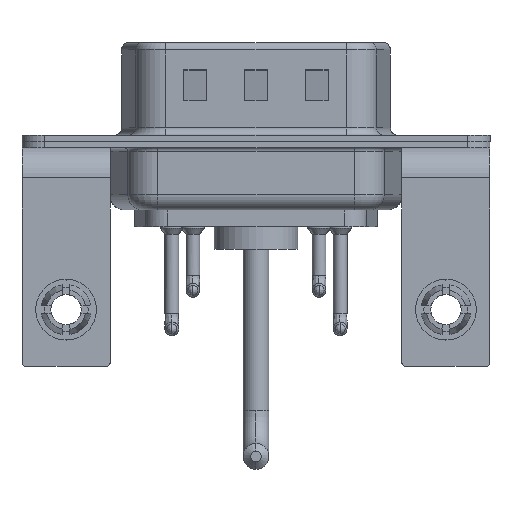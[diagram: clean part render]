
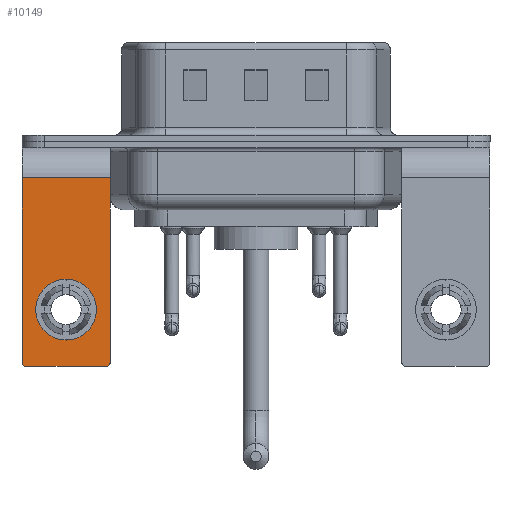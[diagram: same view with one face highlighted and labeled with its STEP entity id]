
A CAD part, front view. The second image highlights one B-rep face of the part: STEP entity #10149.
In plain terms, the highlighted planar face has unit normal (0, -1, 0).
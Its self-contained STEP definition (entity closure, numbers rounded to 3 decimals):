
#185 = DIRECTION ( 'NONE',  ( 0., 0., 1. ) ) ;
#864 = FACE_OUTER_BOUND ( 'NONE', #9699, .T. ) ;
#1735 = DIRECTION ( 'NONE',  ( 0., -1., 0. ) ) ;
#1740 = CARTESIAN_POINT ( 'NONE',  ( 0., -6.25, -11.07 ) ) ;
#1977 = VECTOR ( 'NONE', #4359, 1000. ) ;
#2109 = CARTESIAN_POINT ( 'NONE',  ( -2.65, -6.25, -14.8 ) ) ;
#2122 = DIRECTION ( 'NONE',  ( 0., 1., 0. ) ) ;
#2228 = VECTOR ( 'NONE', #6798, 1000. ) ;
#2247 = EDGE_CURVE ( 'NONE', #16355, #16900, #10989, .T. ) ;
#2508 = CARTESIAN_POINT ( 'NONE',  ( -2.65, -6.25, -14.55 ) ) ;
#2627 = DIRECTION ( 'NONE',  ( 0., 0., 1. ) ) ;
#2643 = CARTESIAN_POINT ( 'NONE',  ( 2.65, -6.25, -14.8 ) ) ;
#2855 = EDGE_CURVE ( 'NONE', #8489, #16174, #4055, .T. ) ;
#3409 = DIRECTION ( 'NONE',  ( 0., 0., 1. ) ) ;
#3524 = VERTEX_POINT ( 'NONE', #2643 ) ;
#4055 = CIRCLE ( 'NONE', #6878, 2. ) ;
#4086 = DIRECTION ( 'NONE',  ( 0., -1., 0. ) ) ;
#4359 = DIRECTION ( 'NONE',  ( -1., 0., 0. ) ) ;
#4450 = DIRECTION ( 'NONE',  ( -1., 0., 0. ) ) ;
#4702 = CARTESIAN_POINT ( 'NONE',  ( -2.9, -6.25, -14.55 ) ) ;
#4952 = VERTEX_POINT ( 'NONE', #2109 ) ;
#5568 = CIRCLE ( 'NONE', #12642, 2. ) ;
#5729 = CARTESIAN_POINT ( 'NONE',  ( -2.9, -6.25, -2.4 ) ) ;
#6011 = LINE ( 'NONE', #12774, #1977 ) ;
#6091 = ORIENTED_EDGE ( 'NONE', *, *, #17905, .F. ) ;
#6798 = DIRECTION ( 'NONE',  ( 0., 0., -1. ) ) ;
#6839 = DIRECTION ( 'NONE',  ( 0., 0., 1. ) ) ;
#6878 = AXIS2_PLACEMENT_3D ( 'NONE', #12440, #2122, #9328 ) ;
#7045 = EDGE_CURVE ( 'NONE', #16174, #8489, #5568, .T. ) ;
#7356 = CIRCLE ( 'NONE', #14770, 0.25 ) ;
#7402 = AXIS2_PLACEMENT_3D ( 'NONE', #2508, #4086, #2627 ) ;
#7835 = DIRECTION ( 'NONE',  ( 0., 1., 0. ) ) ;
#8130 = ORIENTED_EDGE ( 'NONE', *, *, #9040, .T. ) ;
#8357 = LINE ( 'NONE', #21769, #2228 ) ;
#8489 = VERTEX_POINT ( 'NONE', #16019 ) ;
#8699 = EDGE_CURVE ( 'NONE', #14943, #4952, #12011, .T. ) ;
#9040 = EDGE_CURVE ( 'NONE', #3524, #21525, #7356, .T. ) ;
#9328 = DIRECTION ( 'NONE',  ( 0., 0., 1. ) ) ;
#9699 = EDGE_LOOP ( 'NONE', ( #14322, #21461, #6091, #8130, #18547, #20363 ) ) ;
#10149 = ADVANCED_FACE ( 'NONE', ( #16037, #864 ), #19584, .F. ) ;
#10279 = AXIS2_PLACEMENT_3D ( 'NONE', #17918, #7835, #3409 ) ;
#10752 = VECTOR ( 'NONE', #19427, 1000. ) ;
#10989 = LINE ( 'NONE', #17960, #13922 ) ;
#11002 = CARTESIAN_POINT ( 'NONE',  ( 2.9, -6.25, -2.4 ) ) ;
#12011 = CIRCLE ( 'NONE', #7402, 0.25 ) ;
#12153 = CARTESIAN_POINT ( 'NONE',  ( 2.65, -6.25, -14.55 ) ) ;
#12440 = CARTESIAN_POINT ( 'NONE',  ( 0., -6.25, -11.07 ) ) ;
#12642 = AXIS2_PLACEMENT_3D ( 'NONE', #1740, #13589, #6839 ) ;
#12774 = CARTESIAN_POINT ( 'NONE',  ( 2.9, -6.25, -14.8 ) ) ;
#13589 = DIRECTION ( 'NONE',  ( 0., 1., 0. ) ) ;
#13870 = CARTESIAN_POINT ( 'NONE',  ( 2.9, -6.25, -2.4 ) ) ;
#13922 = VECTOR ( 'NONE', #4450, 1000. ) ;
#14322 = ORIENTED_EDGE ( 'NONE', *, *, #15181, .T. ) ;
#14770 = AXIS2_PLACEMENT_3D ( 'NONE', #12153, #1735, #185 ) ;
#14943 = VERTEX_POINT ( 'NONE', #4702 ) ;
#15181 = EDGE_CURVE ( 'NONE', #16900, #14943, #8357, .T. ) ;
#15406 = EDGE_CURVE ( 'NONE', #16355, #21525, #16416, .T. ) ;
#16019 = CARTESIAN_POINT ( 'NONE',  ( 0., -6.25, -9.07 ) ) ;
#16037 = FACE_BOUND ( 'NONE', #21721, .T. ) ;
#16174 = VERTEX_POINT ( 'NONE', #16341 ) ;
#16341 = CARTESIAN_POINT ( 'NONE',  ( 0., -6.25, -13.07 ) ) ;
#16355 = VERTEX_POINT ( 'NONE', #13870 ) ;
#16416 = LINE ( 'NONE', #11002, #10752 ) ;
#16900 = VERTEX_POINT ( 'NONE', #5729 ) ;
#17905 = EDGE_CURVE ( 'NONE', #3524, #4952, #6011, .T. ) ;
#17918 = CARTESIAN_POINT ( 'NONE',  ( 2.9, -6.25, -2.4 ) ) ;
#17960 = CARTESIAN_POINT ( 'NONE',  ( 2.9, -6.25, -2.4 ) ) ;
#18209 = CARTESIAN_POINT ( 'NONE',  ( 2.9, -6.25, -14.55 ) ) ;
#18437 = ORIENTED_EDGE ( 'NONE', *, *, #2855, .T. ) ;
#18547 = ORIENTED_EDGE ( 'NONE', *, *, #15406, .F. ) ;
#19427 = DIRECTION ( 'NONE',  ( 0., 0., -1. ) ) ;
#19584 = PLANE ( 'NONE',  #10279 ) ;
#19619 = ORIENTED_EDGE ( 'NONE', *, *, #7045, .T. ) ;
#20363 = ORIENTED_EDGE ( 'NONE', *, *, #2247, .T. ) ;
#21461 = ORIENTED_EDGE ( 'NONE', *, *, #8699, .T. ) ;
#21525 = VERTEX_POINT ( 'NONE', #18209 ) ;
#21721 = EDGE_LOOP ( 'NONE', ( #19619, #18437 ) ) ;
#21769 = CARTESIAN_POINT ( 'NONE',  ( -2.9, -6.25, -2.4 ) ) ;
